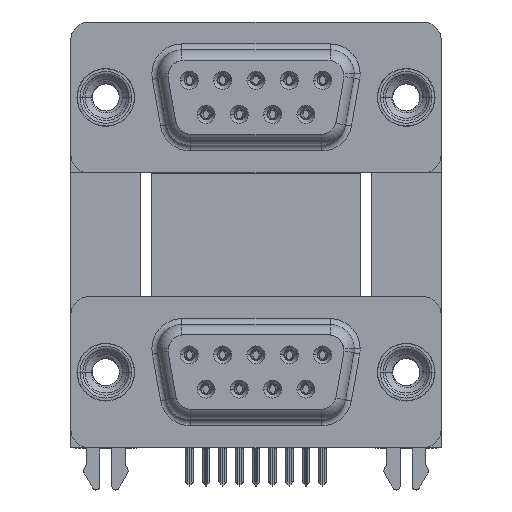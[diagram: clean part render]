
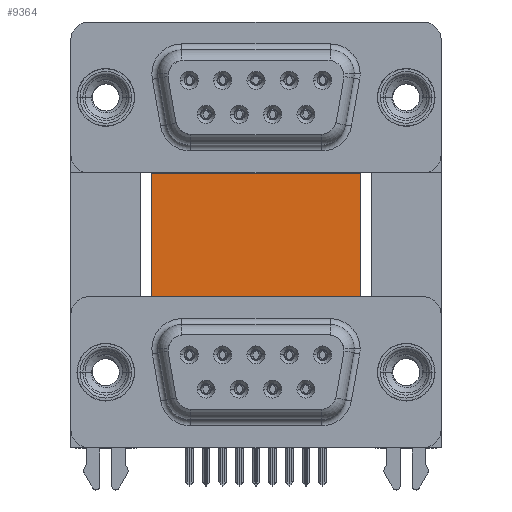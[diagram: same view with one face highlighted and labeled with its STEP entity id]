
A CAD part, top view. The second image highlights one B-rep face of the part: STEP entity #9364.
In plain terms, the highlighted planar face has unit normal (0, 0, 1).
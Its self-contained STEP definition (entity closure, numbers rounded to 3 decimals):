
#348 = VERTEX_POINT ( 'NONE', #38749 ) ;
#450 = CARTESIAN_POINT ( 'NONE',  ( 21.2, -0.735, -12. ) ) ;
#838 = VERTEX_POINT ( 'NONE', #38684 ) ;
#1207 = DIRECTION ( 'NONE',  ( 1., 0., 0. ) ) ;
#1833 = VECTOR ( 'NONE', #2480, 1000. ) ;
#2480 = DIRECTION ( 'NONE',  ( 0., -1., 0. ) ) ;
#2703 = CARTESIAN_POINT ( 'NONE',  ( 3.79, 16.585, -12. ) ) ;
#5176 = VERTEX_POINT ( 'NONE', #26945 ) ;
#5402 = CARTESIAN_POINT ( 'NONE',  ( 2.9, -3.735, -12. ) ) ;
#5533 = EDGE_CURVE ( 'NONE', #838, #25697, #41739, .T. ) ;
#6151 = ORIENTED_EDGE ( 'NONE', *, *, #18669, .F. ) ;
#6330 = VECTOR ( 'NONE', #34016, 1000. ) ;
#6597 = LINE ( 'NONE', #42801, #28808 ) ;
#7029 = ORIENTED_EDGE ( 'NONE', *, *, #41590, .T. ) ;
#8503 = VECTOR ( 'NONE', #32494, 1000. ) ;
#9364 = ADVANCED_FACE ( 'NONE', ( #26227 ), #39347, .F. ) ;
#10256 = DIRECTION ( 'NONE',  ( 1., 0., 0. ) ) ;
#10394 = EDGE_CURVE ( 'NONE', #21963, #5176, #16478, .T. ) ;
#10903 = VECTOR ( 'NONE', #1207, 1000. ) ;
#12583 = VECTOR ( 'NONE', #40306, 1000. ) ;
#12791 = ORIENTED_EDGE ( 'NONE', *, *, #30319, .T. ) ;
#14132 = LINE ( 'NONE', #20776, #10903 ) ;
#16478 = LINE ( 'NONE', #30017, #25702 ) ;
#17133 = VERTEX_POINT ( 'NONE', #34656 ) ;
#17985 = DIRECTION ( 'NONE',  ( -0.336, -0.942, 0. ) ) ;
#18164 = VECTOR ( 'NONE', #17985, 1000. ) ;
#18669 = EDGE_CURVE ( 'NONE', #17133, #40622, #30094, .T. ) ;
#19701 = CARTESIAN_POINT ( 'NONE',  ( 3.79, -0.735, -12. ) ) ;
#20776 = CARTESIAN_POINT ( 'NONE',  ( 3.79, 16.585, -12. ) ) ;
#21527 = LINE ( 'NONE', #25075, #18164 ) ;
#21546 = VERTEX_POINT ( 'NONE', #35811 ) ;
#21963 = VERTEX_POINT ( 'NONE', #22205 ) ;
#22129 = CARTESIAN_POINT ( 'NONE',  ( 22.59, -4.635, -12. ) ) ;
#22205 = CARTESIAN_POINT ( 'NONE',  ( 2.9, -3.735, -12. ) ) ;
#22407 = ORIENTED_EDGE ( 'NONE', *, *, #29328, .T. ) ;
#22448 = CARTESIAN_POINT ( 'NONE',  ( 3.79, 16.585, -12. ) ) ;
#22876 = DIRECTION ( 'NONE',  ( -0.336, 0.942, 0. ) ) ;
#22894 = DIRECTION ( 'NONE',  ( 0., 0., -1. ) ) ;
#22922 = EDGE_CURVE ( 'NONE', #21546, #34833, #30302, .T. ) ;
#23421 = CARTESIAN_POINT ( 'NONE',  ( 21.2, 16.585, -12. ) ) ;
#24432 = CARTESIAN_POINT ( 'NONE',  ( 22.09, -4.635, -12. ) ) ;
#24744 = EDGE_CURVE ( 'NONE', #348, #17133, #14132, .T. ) ;
#24933 = ORIENTED_EDGE ( 'NONE', *, *, #22922, .T. ) ;
#25075 = CARTESIAN_POINT ( 'NONE',  ( 2.4, -4.635, -12. ) ) ;
#25697 = VERTEX_POINT ( 'NONE', #22129 ) ;
#25702 = VECTOR ( 'NONE', #10256, 1000. ) ;
#25765 = LINE ( 'NONE', #38878, #31871 ) ;
#26227 = FACE_OUTER_BOUND ( 'NONE', #39191, .T. ) ;
#26945 = CARTESIAN_POINT ( 'NONE',  ( 22.09, -3.735, -12. ) ) ;
#27406 = CARTESIAN_POINT ( 'NONE',  ( 2.9, -4.635, -12. ) ) ;
#28808 = VECTOR ( 'NONE', #39900, 1000. ) ;
#29149 = ORIENTED_EDGE ( 'NONE', *, *, #10394, .T. ) ;
#29328 = EDGE_CURVE ( 'NONE', #38306, #21546, #21527, .T. ) ;
#30017 = CARTESIAN_POINT ( 'NONE',  ( 3.79, -3.735, -12. ) ) ;
#30094 = LINE ( 'NONE', #23421, #12583 ) ;
#30302 = LINE ( 'NONE', #27406, #34898 ) ;
#30319 = EDGE_CURVE ( 'NONE', #348, #38306, #32924, .T. ) ;
#30669 = ORIENTED_EDGE ( 'NONE', *, *, #31122, .T. ) ;
#31122 = EDGE_CURVE ( 'NONE', #5176, #838, #6597, .T. ) ;
#31871 = VECTOR ( 'NONE', #22876, 1000. ) ;
#32494 = DIRECTION ( 'NONE',  ( 0., 1., 0. ) ) ;
#32924 = LINE ( 'NONE', #2703, #1833 ) ;
#34016 = DIRECTION ( 'NONE',  ( 1., 0., 0. ) ) ;
#34656 = CARTESIAN_POINT ( 'NONE',  ( 21.2, 16.585, -12. ) ) ;
#34833 = VERTEX_POINT ( 'NONE', #35658 ) ;
#34898 = VECTOR ( 'NONE', #43855, 1000. ) ;
#35658 = CARTESIAN_POINT ( 'NONE',  ( 2.9, -4.635, -12. ) ) ;
#35811 = CARTESIAN_POINT ( 'NONE',  ( 2.4, -4.635, -12. ) ) ;
#35813 = LINE ( 'NONE', #5402, #8503 ) ;
#35838 = EDGE_CURVE ( 'NONE', #34833, #21963, #35813, .T. ) ;
#36241 = ORIENTED_EDGE ( 'NONE', *, *, #5533, .T. ) ;
#36448 = DIRECTION ( 'NONE',  ( -1., 0., 0. ) ) ;
#38306 = VERTEX_POINT ( 'NONE', #19701 ) ;
#38684 = CARTESIAN_POINT ( 'NONE',  ( 22.09, -4.635, -12. ) ) ;
#38749 = CARTESIAN_POINT ( 'NONE',  ( 3.79, 16.585, -12. ) ) ;
#38878 = CARTESIAN_POINT ( 'NONE',  ( 22.59, -4.635, -12. ) ) ;
#39191 = EDGE_LOOP ( 'NONE', ( #29149, #30669, #36241, #7029, #6151, #41986, #12791, #22407, #24933, #39297 ) ) ;
#39297 = ORIENTED_EDGE ( 'NONE', *, *, #35838, .T. ) ;
#39347 = PLANE ( 'NONE',  #40550 ) ;
#39900 = DIRECTION ( 'NONE',  ( 0., -1., 0. ) ) ;
#40306 = DIRECTION ( 'NONE',  ( 0., -1., 0. ) ) ;
#40550 = AXIS2_PLACEMENT_3D ( 'NONE', #22448, #22894, #36448 ) ;
#40622 = VERTEX_POINT ( 'NONE', #450 ) ;
#41590 = EDGE_CURVE ( 'NONE', #25697, #40622, #25765, .T. ) ;
#41739 = LINE ( 'NONE', #24432, #6330 ) ;
#41986 = ORIENTED_EDGE ( 'NONE', *, *, #24744, .F. ) ;
#42801 = CARTESIAN_POINT ( 'NONE',  ( 22.09, -3.735, -12. ) ) ;
#43855 = DIRECTION ( 'NONE',  ( 1., 0., 0. ) ) ;
